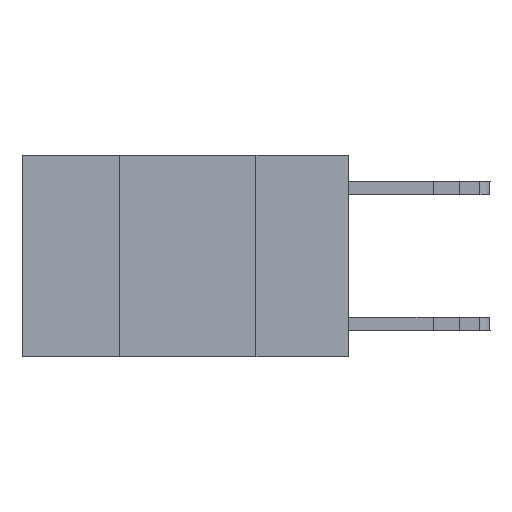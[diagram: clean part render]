
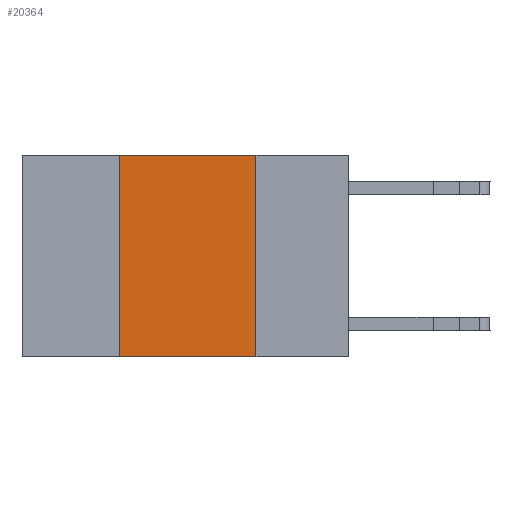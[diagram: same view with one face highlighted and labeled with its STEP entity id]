
A CAD part, left-side view. The second image highlights one B-rep face of the part: STEP entity #20364.
In plain terms, the highlighted planar face has unit normal (-1, 0, 0).
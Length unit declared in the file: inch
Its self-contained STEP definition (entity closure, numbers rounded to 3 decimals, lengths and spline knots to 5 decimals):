
#363 = DIRECTION ( 'NONE',  ( 0., -1., 0. ) ) ;
#846 = ORIENTED_EDGE ( 'NONE', *, *, #5972, .F. ) ;
#883 = ORIENTED_EDGE ( 'NONE', *, *, #2687, .F. ) ;
#2438 = VECTOR ( 'NONE', #8216, 39.37008 ) ;
#2629 = DIRECTION ( 'NONE',  ( 0., 0., 1. ) ) ;
#2687 = EDGE_CURVE ( 'NONE', #2699, #21650, #8037, .T. ) ;
#2699 = VERTEX_POINT ( 'NONE', #17935 ) ;
#3931 = DIRECTION ( 'NONE',  ( 1., 0., 0. ) ) ;
#4568 = VECTOR ( 'NONE', #2629, 39.37008 ) ;
#5056 = ORIENTED_EDGE ( 'NONE', *, *, #5335, .T. ) ;
#5335 = EDGE_CURVE ( 'NONE', #2699, #18675, #20251, .T. ) ;
#5452 = CARTESIAN_POINT ( 'NONE',  ( 0., 0.17, 0. ) ) ;
#5474 = LINE ( 'NONE', #20550, #14178 ) ;
#5972 = EDGE_CURVE ( 'NONE', #14835, #18675, #5474, .T. ) ;
#6167 = AXIS2_PLACEMENT_3D ( 'NONE', #15886, #3931, #12169 ) ;
#7186 = ORIENTED_EDGE ( 'NONE', *, *, #21272, .F. ) ;
#8037 = LINE ( 'NONE', #12874, #4568 ) ;
#8149 = EDGE_LOOP ( 'NONE', ( #846, #7186, #883, #5056 ) ) ;
#8216 = DIRECTION ( 'NONE',  ( 0., -1., 0. ) ) ;
#8365 = CARTESIAN_POINT ( 'NONE',  ( 0., 0.42, 0. ) ) ;
#10417 = DIRECTION ( 'NONE',  ( 0., 0., -1. ) ) ;
#10473 = PLANE ( 'NONE',  #6167 ) ;
#10608 = CARTESIAN_POINT ( 'NONE',  ( 0., 0.6, 0. ) ) ;
#12169 = DIRECTION ( 'NONE',  ( 0., 0., -1. ) ) ;
#12874 = CARTESIAN_POINT ( 'NONE',  ( 0., 0.42, 0. ) ) ;
#13848 = FACE_OUTER_BOUND ( 'NONE', #8149, .T. ) ;
#14178 = VECTOR ( 'NONE', #10417, 39.37008 ) ;
#14835 = VERTEX_POINT ( 'NONE', #5452 ) ;
#15802 = LINE ( 'NONE', #10608, #16264 ) ;
#15886 = CARTESIAN_POINT ( 'NONE',  ( 0., 0.6, 0. ) ) ;
#16264 = VECTOR ( 'NONE', #363, 39.37008 ) ;
#16664 = CARTESIAN_POINT ( 'NONE',  ( 0., 0.6, -0.37 ) ) ;
#17935 = CARTESIAN_POINT ( 'NONE',  ( 0., 0.42, -0.37 ) ) ;
#18675 = VERTEX_POINT ( 'NONE', #21361 ) ;
#20251 = LINE ( 'NONE', #16664, #2438 ) ;
#20364 = ADVANCED_FACE ( 'NONE', ( #13848 ), #10473, .F. ) ;
#20550 = CARTESIAN_POINT ( 'NONE',  ( 0., 0.17, 0. ) ) ;
#21272 = EDGE_CURVE ( 'NONE', #21650, #14835, #15802, .T. ) ;
#21361 = CARTESIAN_POINT ( 'NONE',  ( 0., 0.17, -0.37 ) ) ;
#21650 = VERTEX_POINT ( 'NONE', #8365 ) ;
